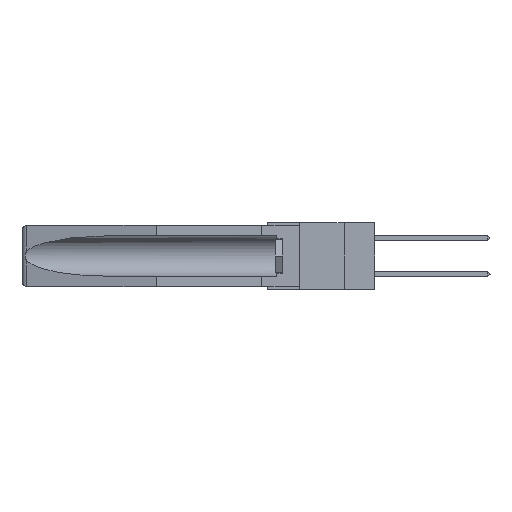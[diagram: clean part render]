
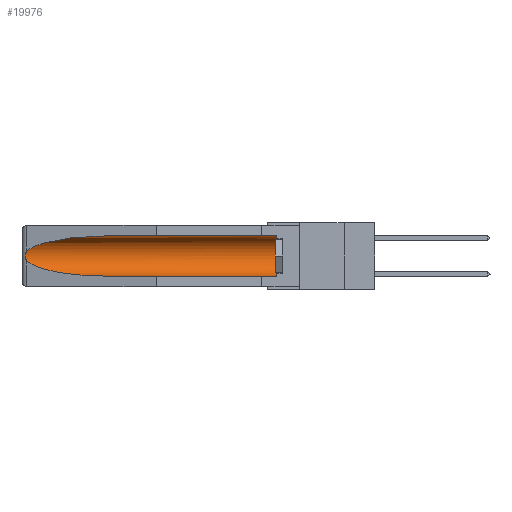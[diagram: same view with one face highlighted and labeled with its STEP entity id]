
A CAD part, left-side view. The second image highlights one B-rep face of the part: STEP entity #19976.
In plain terms, the highlighted cylindrical face has radius 2.857 mm (diameter 5.715 mm), a partial arc.
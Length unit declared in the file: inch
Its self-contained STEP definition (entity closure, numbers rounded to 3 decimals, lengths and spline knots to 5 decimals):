
#629 = EDGE_CURVE ( 'NONE', #20806, #24908, #1855, .T. ) ;
#1358 = CARTESIAN_POINT ( 'NONE',  ( 0.2675, 1.53308, -0.16763 ) ) ;
#1384 = CARTESIAN_POINT ( 'NONE',  ( 0.155, 1.07973, -0.284 ) ) ;
#1502 = CARTESIAN_POINT ( 'NONE',  ( 0.155, 0.126, -0.059 ) ) ;
#1576 = DIRECTION ( 'NONE',  ( 0., -1., 0. ) ) ;
#1799 = CYLINDRICAL_SURFACE ( 'NONE', #8014, 0.1125 ) ;
#1855 = B_SPLINE_CURVE_WITH_KNOTS ( 'NONE', 3,
 ( #27247, #18647, #12199, #27339, #1358, #3558, #25528, #12671, #12396, #27791 ),
 .UNSPECIFIED., .F., .F.,
 ( 4, 2, 2, 2, 4 ),
 ( 0., 0.00029, 0.00058, 0.00087, 0.00117 ),
 .UNSPECIFIED. ) ;
#2433 = EDGE_CURVE ( 'NONE', #24908, #10611, #25675, .T. ) ;
#3473 = EDGE_CURVE ( 'NONE', #16794, #20806, #20691, .T. ) ;
#3558 = CARTESIAN_POINT ( 'NONE',  ( 0.2675, 1.53308, -0.17534 ) ) ;
#4967 = VECTOR ( 'NONE', #19041, 39.37008 ) ;
#5115 = VERTEX_POINT ( 'NONE', #1502 ) ;
#5968 = LINE ( 'NONE', #27652, #4967 ) ;
#7522 = CARTESIAN_POINT ( 'NONE',  ( 0.155, 1.07973, -0.059 ) ) ;
#7798 = CARTESIAN_POINT ( 'NONE',  ( 0.26537, 1.52718, -0.14972 ) ) ;
#7878 = DIRECTION ( 'NONE',  ( 0., 1., 0. ) ) ;
#8014 = AXIS2_PLACEMENT_3D ( 'NONE', #20876, #7878, #10076 ) ;
#8410 = ORIENTED_EDGE ( 'NONE', *, *, #2433, .T. ) ;
#9492 = AXIS2_PLACEMENT_3D ( 'NONE', #16942, #1576, #23128 ) ;
#10004 = CIRCLE ( 'NONE', #9492, 0.1125 ) ;
#10076 = DIRECTION ( 'NONE',  ( 0., 0., 1. ) ) ;
#10490 = ORIENTED_EDGE ( 'NONE', *, *, #3473, .T. ) ;
#10579 = ORIENTED_EDGE ( 'NONE', *, *, #14862, .F. ) ;
#10611 = VERTEX_POINT ( 'NONE', #17139 ) ;
#12199 = CARTESIAN_POINT ( 'NONE',  ( 0.26654, 1.53092, -0.15636 ) ) ;
#12396 = CARTESIAN_POINT ( 'NONE',  ( 0.26597, 1.5296, -0.19026 ) ) ;
#12671 = CARTESIAN_POINT ( 'NONE',  ( 0.26655, 1.53094, -0.18657 ) ) ;
#14134 = CARTESIAN_POINT ( 'NONE',  ( 0.21114, 1.30732, -0.284 ) ) ;
#14317 = CARTESIAN_POINT ( 'NONE',  ( 0.26537, 1.52718, -0.19328 ) ) ;
#14624 = CARTESIAN_POINT ( 'NONE',  ( 0.155, 0.126, -0.284 ) ) ;
#14862 = EDGE_CURVE ( 'NONE', #15310, #10611, #19294, .T. ) ;
#15310 = VERTEX_POINT ( 'NONE', #14624 ) ;
#16412 = EDGE_LOOP ( 'NONE', ( #10490, #19661, #8410, #10579, #26351, #21787 ) ) ;
#16794 = VERTEX_POINT ( 'NONE', #7522 ) ;
#16942 = CARTESIAN_POINT ( 'NONE',  ( 0.155, 0.126, -0.1715 ) ) ;
#17000 = CARTESIAN_POINT ( 'NONE',  ( 0.26537, 1.52718, -0.14972 ) ) ;
#17139 = CARTESIAN_POINT ( 'NONE',  ( 0.155, 1.07973, -0.284 ) ) ;
#17895 = CARTESIAN_POINT ( 'NONE',  ( 0.155, -0.30754, -0.284 ) ) ;
#18647 = CARTESIAN_POINT ( 'NONE',  ( 0.26597, 1.52961, -0.15275 ) ) ;
#19041 = DIRECTION ( 'NONE',  ( 0., 1., 0. ) ) ;
#19294 = LINE ( 'NONE', #17895, #24038 ) ;
#19661 = ORIENTED_EDGE ( 'NONE', *, *, #629, .T. ) ;
#19976 = ADVANCED_FACE ( 'NONE', ( #20843 ), #1799, .F. ) ;
#20019 = EDGE_CURVE ( 'NONE', #15310, #5115, #10004, .T. ) ;
#20436 = CARTESIAN_POINT ( 'NONE',  ( 0.21114, 1.30732, -0.059 ) ) ;
#20691 =( BOUNDED_CURVE ( )  B_SPLINE_CURVE ( 3, ( #20804, #20436, #24953, #7798 ),
 .UNSPECIFIED., .F., .T. ) 
 B_SPLINE_CURVE_WITH_KNOTS ( ( 4, 4 ),
 ( 4.71239, 6.08839 ),
 .UNSPECIFIED. ) 
 CURVE ( )  GEOMETRIC_REPRESENTATION_ITEM ( )  RATIONAL_B_SPLINE_CURVE ( ( 1., 0.848, 0.848, 1. ) ) 
 REPRESENTATION_ITEM ( '' )  );
#20804 = CARTESIAN_POINT ( 'NONE',  ( 0.155, 1.07973, -0.059 ) ) ;
#20806 = VERTEX_POINT ( 'NONE', #17000 ) ;
#20843 = FACE_OUTER_BOUND ( 'NONE', #16412, .T. ) ;
#20876 = CARTESIAN_POINT ( 'NONE',  ( 0.155, -0.30754, -0.1715 ) ) ;
#21787 = ORIENTED_EDGE ( 'NONE', *, *, #25423, .T. ) ;
#22077 = DIRECTION ( 'NONE',  ( 0., 1., 0. ) ) ;
#23128 = DIRECTION ( 'NONE',  ( 0., 0., 1. ) ) ;
#23439 = CARTESIAN_POINT ( 'NONE',  ( 0.26537, 1.52718, -0.19328 ) ) ;
#24038 = VECTOR ( 'NONE', #22077, 39.37008 ) ;
#24908 = VERTEX_POINT ( 'NONE', #23439 ) ;
#24953 = CARTESIAN_POINT ( 'NONE',  ( 0.25451, 1.48313, -0.09465 ) ) ;
#25423 = EDGE_CURVE ( 'NONE', #5115, #16794, #5968, .T. ) ;
#25528 = CARTESIAN_POINT ( 'NONE',  ( 0.2673, 1.53269, -0.17917 ) ) ;
#25675 =( BOUNDED_CURVE ( )  B_SPLINE_CURVE ( 3, ( #14317, #27082, #14134, #1384 ),
 .UNSPECIFIED., .F., .F. ) 
 B_SPLINE_CURVE_WITH_KNOTS ( ( 4, 4 ),
 ( 0.1948, 1.5708 ),
 .UNSPECIFIED. ) 
 CURVE ( )  GEOMETRIC_REPRESENTATION_ITEM ( )  RATIONAL_B_SPLINE_CURVE ( ( 1., 0.848, 0.848, 1. ) ) 
 REPRESENTATION_ITEM ( '' )  );
#26351 = ORIENTED_EDGE ( 'NONE', *, *, #20019, .T. ) ;
#27082 = CARTESIAN_POINT ( 'NONE',  ( 0.25451, 1.48313, -0.24835 ) ) ;
#27247 = CARTESIAN_POINT ( 'NONE',  ( 0.26537, 1.52718, -0.14972 ) ) ;
#27339 = CARTESIAN_POINT ( 'NONE',  ( 0.2673, 1.5327, -0.16383 ) ) ;
#27652 = CARTESIAN_POINT ( 'NONE',  ( 0.155, -0.30754, -0.059 ) ) ;
#27791 = CARTESIAN_POINT ( 'NONE',  ( 0.26537, 1.52718, -0.19328 ) ) ;
